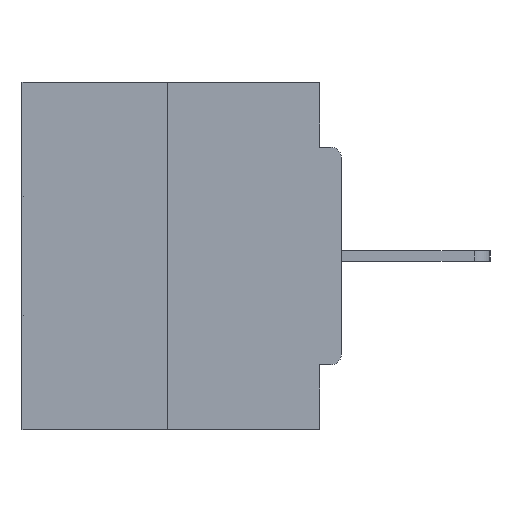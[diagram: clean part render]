
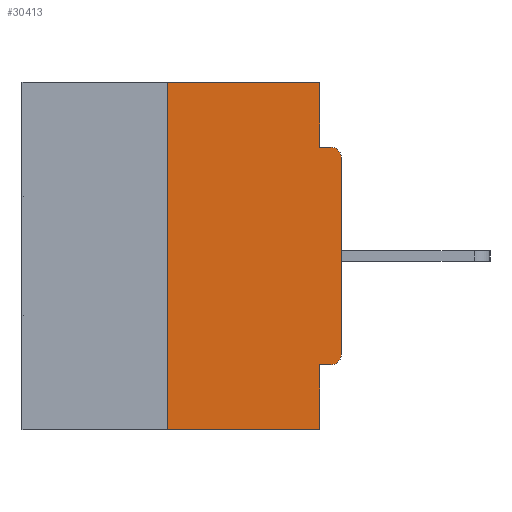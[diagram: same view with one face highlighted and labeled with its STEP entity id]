
A CAD part, left-side view. The second image highlights one B-rep face of the part: STEP entity #30413.
In plain terms, the highlighted planar face has unit normal (-1, 0, 0).
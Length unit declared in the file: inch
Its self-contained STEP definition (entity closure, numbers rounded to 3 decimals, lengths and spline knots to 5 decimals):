
#160 = CARTESIAN_POINT ( 'NONE',  ( 0., 0.015, -0.3915 ) ) ;
#315 = LINE ( 'NONE', #8614, #19158 ) ;
#736 = EDGE_LOOP ( 'NONE', ( #5084, #3378, #30327, #10362, #2098, #21976, #33199, #26972, #2705, #9824 ) ) ;
#741 = CARTESIAN_POINT ( 'NONE',  ( 0., 0.46, 0. ) ) ;
#1181 = VERTEX_POINT ( 'NONE', #21905 ) ;
#1858 = VERTEX_POINT ( 'NONE', #15717 ) ;
#1871 = VERTEX_POINT ( 'NONE', #31668 ) ;
#2098 = ORIENTED_EDGE ( 'NONE', *, *, #7932, .F. ) ;
#2479 = VERTEX_POINT ( 'NONE', #21186 ) ;
#2517 = FACE_OUTER_BOUND ( 'NONE', #736, .T. ) ;
#2705 = ORIENTED_EDGE ( 'NONE', *, *, #33017, .F. ) ;
#3022 = DIRECTION ( 'NONE',  ( 0., 0., -1. ) ) ;
#3031 = DIRECTION ( 'NONE',  ( 0., 0., -1. ) ) ;
#3331 = CIRCLE ( 'NONE', #6599, 0.015 ) ;
#3378 = ORIENTED_EDGE ( 'NONE', *, *, #6196, .F. ) ;
#3717 = LINE ( 'NONE', #26594, #18705 ) ;
#3879 = CARTESIAN_POINT ( 'NONE',  ( 0., 0., 0. ) ) ;
#4012 = VECTOR ( 'NONE', #5627, 39.37008 ) ;
#5084 = ORIENTED_EDGE ( 'NONE', *, *, #21192, .F. ) ;
#5627 = DIRECTION ( 'NONE',  ( 0., -1., 0. ) ) ;
#6196 = EDGE_CURVE ( 'NONE', #30437, #15822, #3717, .T. ) ;
#6567 = EDGE_CURVE ( 'NONE', #1858, #1871, #29551, .T. ) ;
#6599 = AXIS2_PLACEMENT_3D ( 'NONE', #32245, #12194, #32912 ) ;
#6944 = EDGE_CURVE ( 'NONE', #30437, #13059, #15191, .T. ) ;
#6996 = CARTESIAN_POINT ( 'NONE',  ( 0., 0.25, 0. ) ) ;
#7932 = EDGE_CURVE ( 'NONE', #1858, #8710, #11027, .T. ) ;
#8077 = DIRECTION ( 'NONE',  ( 0., -1., 0. ) ) ;
#8165 = CARTESIAN_POINT ( 'NONE',  ( 0., 0., -0.0935 ) ) ;
#8614 = CARTESIAN_POINT ( 'NONE',  ( 0., 0.031, -0.5 ) ) ;
#8710 = VERTEX_POINT ( 'NONE', #21254 ) ;
#9824 = ORIENTED_EDGE ( 'NONE', *, *, #21963, .F. ) ;
#9939 = CARTESIAN_POINT ( 'NONE',  ( 0., 0.031, 0. ) ) ;
#10362 = ORIENTED_EDGE ( 'NONE', *, *, #20417, .F. ) ;
#10770 = VERTEX_POINT ( 'NONE', #18094 ) ;
#10873 = LINE ( 'NONE', #8165, #4012 ) ;
#11027 = LINE ( 'NONE', #21379, #16603 ) ;
#11274 = VECTOR ( 'NONE', #21344, 39.37008 ) ;
#12194 = DIRECTION ( 'NONE',  ( -1., 0., 0. ) ) ;
#13059 = VERTEX_POINT ( 'NONE', #19005 ) ;
#13258 = AXIS2_PLACEMENT_3D ( 'NONE', #160, #26244, #3031 ) ;
#14044 = DIRECTION ( 'NONE',  ( 0., 0., 1. ) ) ;
#15060 = CARTESIAN_POINT ( 'NONE',  ( 0., 0.25, -0.5 ) ) ;
#15191 = LINE ( 'NONE', #31318, #19814 ) ;
#15717 = CARTESIAN_POINT ( 'NONE',  ( 0., 0.015, -0.4065 ) ) ;
#15822 = VERTEX_POINT ( 'NONE', #6996 ) ;
#16603 = VECTOR ( 'NONE', #23592, 39.37008 ) ;
#18094 = CARTESIAN_POINT ( 'NONE',  ( 0., 0.031, -0.0935 ) ) ;
#18454 = EDGE_CURVE ( 'NONE', #21538, #1181, #3331, .T. ) ;
#18705 = VECTOR ( 'NONE', #14044, 39.37008 ) ;
#19005 = CARTESIAN_POINT ( 'NONE',  ( 0., 0.031, -0.5 ) ) ;
#19158 = VECTOR ( 'NONE', #3022, 39.37008 ) ;
#19814 = VECTOR ( 'NONE', #8077, 39.37008 ) ;
#20162 = CARTESIAN_POINT ( 'NONE',  ( 0., 0.46, 0. ) ) ;
#20368 = CARTESIAN_POINT ( 'NONE',  ( 0., 0., -0.1085 ) ) ;
#20417 = EDGE_CURVE ( 'NONE', #8710, #13059, #315, .T. ) ;
#21186 = CARTESIAN_POINT ( 'NONE',  ( 0., 0.031, 0. ) ) ;
#21192 = EDGE_CURVE ( 'NONE', #15822, #2479, #23452, .T. ) ;
#21254 = CARTESIAN_POINT ( 'NONE',  ( 0., 0.031, -0.4065 ) ) ;
#21344 = DIRECTION ( 'NONE',  ( 0., 0., 1. ) ) ;
#21379 = CARTESIAN_POINT ( 'NONE',  ( 0., 0., -0.4065 ) ) ;
#21538 = VERTEX_POINT ( 'NONE', #20368 ) ;
#21905 = CARTESIAN_POINT ( 'NONE',  ( 0., 0.015, -0.0935 ) ) ;
#21963 = EDGE_CURVE ( 'NONE', #2479, #10770, #25384, .T. ) ;
#21976 = ORIENTED_EDGE ( 'NONE', *, *, #6567, .T. ) ;
#23218 = PLANE ( 'NONE',  #33223 ) ;
#23378 = DIRECTION ( 'NONE',  ( 1., 0., 0. ) ) ;
#23452 = LINE ( 'NONE', #741, #30474 ) ;
#23592 = DIRECTION ( 'NONE',  ( 0., 1., 0. ) ) ;
#25384 = LINE ( 'NONE', #9939, #29965 ) ;
#26244 = DIRECTION ( 'NONE',  ( -1., 0., 0. ) ) ;
#26318 = DIRECTION ( 'NONE',  ( 0., -1., 0. ) ) ;
#26594 = CARTESIAN_POINT ( 'NONE',  ( 0., 0.25, 0. ) ) ;
#26972 = ORIENTED_EDGE ( 'NONE', *, *, #18454, .T. ) ;
#28493 = EDGE_CURVE ( 'NONE', #1871, #21538, #31871, .T. ) ;
#29551 = CIRCLE ( 'NONE', #13258, 0.015 ) ;
#29965 = VECTOR ( 'NONE', #33518, 39.37008 ) ;
#30327 = ORIENTED_EDGE ( 'NONE', *, *, #6944, .T. ) ;
#30413 = ADVANCED_FACE ( 'NONE', ( #2517 ), #23218, .F. ) ;
#30437 = VERTEX_POINT ( 'NONE', #15060 ) ;
#30474 = VECTOR ( 'NONE', #26318, 39.37008 ) ;
#30502 = DIRECTION ( 'NONE',  ( 0., 0., -1. ) ) ;
#31318 = CARTESIAN_POINT ( 'NONE',  ( 0., 0.46, -0.5 ) ) ;
#31668 = CARTESIAN_POINT ( 'NONE',  ( 0., 0., -0.3915 ) ) ;
#31871 = LINE ( 'NONE', #3879, #11274 ) ;
#32245 = CARTESIAN_POINT ( 'NONE',  ( 0., 0.015, -0.1085 ) ) ;
#32912 = DIRECTION ( 'NONE',  ( 0., 0., -1. ) ) ;
#33017 = EDGE_CURVE ( 'NONE', #10770, #1181, #10873, .T. ) ;
#33199 = ORIENTED_EDGE ( 'NONE', *, *, #28493, .T. ) ;
#33223 = AXIS2_PLACEMENT_3D ( 'NONE', #20162, #23378, #30502 ) ;
#33518 = DIRECTION ( 'NONE',  ( 0., 0., -1. ) ) ;
